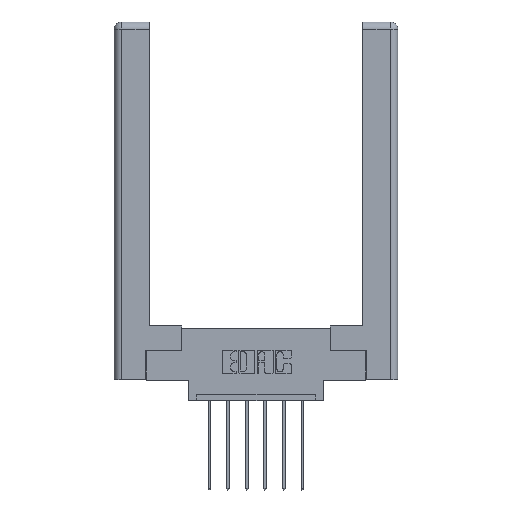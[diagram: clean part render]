
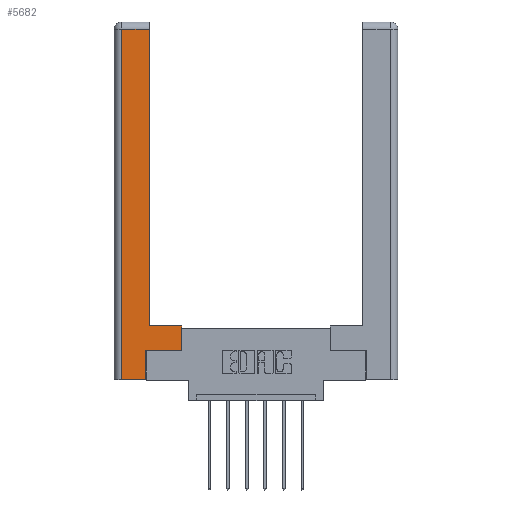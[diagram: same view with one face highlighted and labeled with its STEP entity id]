
A CAD part, top view. The second image highlights one B-rep face of the part: STEP entity #5682.
In plain terms, the highlighted planar face has unit normal (0, 0, 1).
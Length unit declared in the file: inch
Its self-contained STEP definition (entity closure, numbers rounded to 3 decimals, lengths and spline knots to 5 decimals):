
#215 = CARTESIAN_POINT ( 'NONE',  ( 0.265, 0., 0. ) ) ;
#247 = EDGE_CURVE ( 'NONE', #2988, #6720, #2708, .T. ) ;
#294 = CARTESIAN_POINT ( 'NONE',  ( 0.265, 0., 0. ) ) ;
#500 = LINE ( 'NONE', #3402, #3958 ) ;
#581 = CARTESIAN_POINT ( 'NONE',  ( 0.265, 0.245, 0. ) ) ;
#773 = LINE ( 'NONE', #6655, #11834 ) ;
#1253 = LINE ( 'NONE', #3643, #4746 ) ;
#1472 = VERTEX_POINT ( 'NONE', #4372 ) ;
#1591 = EDGE_CURVE ( 'NONE', #9265, #2988, #1253, .T. ) ;
#1894 = DIRECTION ( 'NONE',  ( -1., 0., 0. ) ) ;
#1898 = VECTOR ( 'NONE', #4827, 39.37008 ) ;
#2358 = LINE ( 'NONE', #6507, #5116 ) ;
#2466 = LINE ( 'NONE', #215, #1898 ) ;
#2708 = LINE ( 'NONE', #10089, #6333 ) ;
#2745 = FACE_OUTER_BOUND ( 'NONE', #3810, .T. ) ;
#2988 = VERTEX_POINT ( 'NONE', #7156 ) ;
#3096 = DIRECTION ( 'NONE',  ( 0., 0., -1. ) ) ;
#3133 = CARTESIAN_POINT ( 'NONE',  ( 0.565, 0.245, 0. ) ) ;
#3352 = CARTESIAN_POINT ( 'NONE',  ( 0.0615, 2.94, 0. ) ) ;
#3402 = CARTESIAN_POINT ( 'NONE',  ( 0.0615, 0., 0. ) ) ;
#3560 = DIRECTION ( 'NONE',  ( 0., 1., 0. ) ) ;
#3622 = ORIENTED_EDGE ( 'NONE', *, *, #9724, .T. ) ;
#3643 = CARTESIAN_POINT ( 'NONE',  ( 0.565, 0.45, 0. ) ) ;
#3647 = ORIENTED_EDGE ( 'NONE', *, *, #8527, .T. ) ;
#3667 = VERTEX_POINT ( 'NONE', #581 ) ;
#3810 = EDGE_LOOP ( 'NONE', ( #4378, #9385, #3647, #6621, #10258, #3622, #10993, #5947 ) ) ;
#3958 = VECTOR ( 'NONE', #8896, 39.37008 ) ;
#4372 = CARTESIAN_POINT ( 'NONE',  ( 0.295, 2.94, 0. ) ) ;
#4378 = ORIENTED_EDGE ( 'NONE', *, *, #8846, .T. ) ;
#4746 = VECTOR ( 'NONE', #3560, 39.37008 ) ;
#4827 = DIRECTION ( 'NONE',  ( 1., 0., 0. ) ) ;
#4855 = EDGE_CURVE ( 'NONE', #1472, #10828, #773, .T. ) ;
#5053 = EDGE_CURVE ( 'NONE', #9398, #8965, #2466, .T. ) ;
#5116 = VECTOR ( 'NONE', #7356, 39.37008 ) ;
#5682 = ADVANCED_FACE ( 'NONE', ( #2745 ), #6763, .F. ) ;
#5776 = DIRECTION ( 'NONE',  ( 1., 0., 0. ) ) ;
#5947 = ORIENTED_EDGE ( 'NONE', *, *, #247, .T. ) ;
#6301 = CARTESIAN_POINT ( 'NONE',  ( 0.565, 0.245, 0. ) ) ;
#6333 = VECTOR ( 'NONE', #9174, 39.37008 ) ;
#6507 = CARTESIAN_POINT ( 'NONE',  ( 0.295, 3., 0. ) ) ;
#6572 = LINE ( 'NONE', #10507, #10314 ) ;
#6621 = ORIENTED_EDGE ( 'NONE', *, *, #5053, .T. ) ;
#6623 = CARTESIAN_POINT ( 'NONE',  ( 0.295, 0.45, 0. ) ) ;
#6655 = CARTESIAN_POINT ( 'NONE',  ( 0.0615, 2.94, 0. ) ) ;
#6720 = VERTEX_POINT ( 'NONE', #6623 ) ;
#6763 = PLANE ( 'NONE',  #7414 ) ;
#6808 = VECTOR ( 'NONE', #5776, 39.37008 ) ;
#7156 = CARTESIAN_POINT ( 'NONE',  ( 0.565, 0.45, 0. ) ) ;
#7298 = CARTESIAN_POINT ( 'NONE',  ( 0.0615, 0., 0. ) ) ;
#7356 = DIRECTION ( 'NONE',  ( 0., 1., 0. ) ) ;
#7414 = AXIS2_PLACEMENT_3D ( 'NONE', #7801, #3096, #7695 ) ;
#7695 = DIRECTION ( 'NONE',  ( -1., 0., 0. ) ) ;
#7801 = CARTESIAN_POINT ( 'NONE',  ( 0., 0., 0. ) ) ;
#7893 = EDGE_CURVE ( 'NONE', #8965, #3667, #6572, .T. ) ;
#8527 = EDGE_CURVE ( 'NONE', #10828, #9398, #500, .T. ) ;
#8626 = DIRECTION ( 'NONE',  ( 0., 1., 0. ) ) ;
#8846 = EDGE_CURVE ( 'NONE', #6720, #1472, #2358, .T. ) ;
#8896 = DIRECTION ( 'NONE',  ( 0., -1., 0. ) ) ;
#8965 = VERTEX_POINT ( 'NONE', #294 ) ;
#9174 = DIRECTION ( 'NONE',  ( -1., 0., 0. ) ) ;
#9265 = VERTEX_POINT ( 'NONE', #6301 ) ;
#9385 = ORIENTED_EDGE ( 'NONE', *, *, #4855, .T. ) ;
#9398 = VERTEX_POINT ( 'NONE', #7298 ) ;
#9549 = LINE ( 'NONE', #3133, #6808 ) ;
#9724 = EDGE_CURVE ( 'NONE', #3667, #9265, #9549, .T. ) ;
#10089 = CARTESIAN_POINT ( 'NONE',  ( 0.295, 0.45, 0. ) ) ;
#10258 = ORIENTED_EDGE ( 'NONE', *, *, #7893, .T. ) ;
#10314 = VECTOR ( 'NONE', #8626, 39.37008 ) ;
#10507 = CARTESIAN_POINT ( 'NONE',  ( 0.265, 0.245, 0. ) ) ;
#10828 = VERTEX_POINT ( 'NONE', #3352 ) ;
#10993 = ORIENTED_EDGE ( 'NONE', *, *, #1591, .T. ) ;
#11834 = VECTOR ( 'NONE', #1894, 39.37008 ) ;
